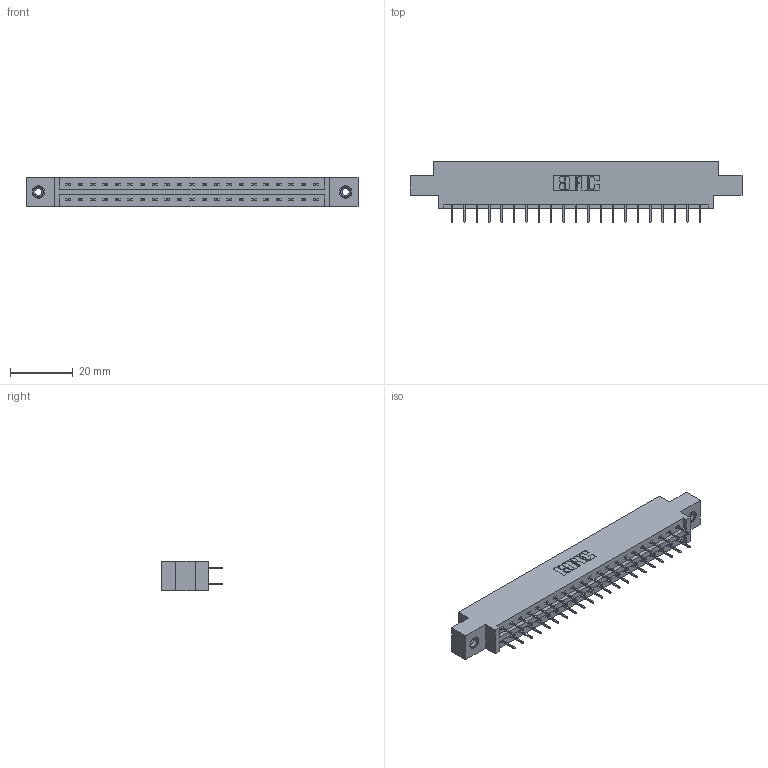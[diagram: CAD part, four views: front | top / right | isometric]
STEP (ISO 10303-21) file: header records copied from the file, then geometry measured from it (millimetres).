
FILE_DESCRIPTION (( 'STEP AP203' ), '1' );
FILE_NAME ('387-042-524-808.STEP', '2018-09-19T22:20:34', ( '' ), ( '' ), 'SwSTEP 2.0', 'SolidWorks 2016', '' );
FILE_SCHEMA (( 'CONFIG_CONTROL_DESIGN' ));
Length unit declared in the file: inch
Products named in the file (4): 387-042-524-808; 337 Part_0.170 Offset - 0.156 Dia-TI; 345-292-001_345-293-124; 345-250-001_345-250-003-102
Assembly tree (45 placements, depth 2):
  387-042-524-808
    337 Part_0.170 Offset - 0.156 Dia-TI
    345-292-001_345-293-124  x42
    345-250-001_345-250-003-102  x2
Bounding box: 106.22 x 19.69 x 9.4 mm (x, y, z)
Volume: 10727.5 mm3; surface area: 11858.4 mm2
Topology: 45 solids, 45 shells, 2614 faces, 7389 edges, 4750 vertices
Faces by surface type: plane 1954, cylinder 644, cone 12, torus 4
Entity records: 20390 total; most frequent: CARTESIAN_POINT 3433, ORIENTED_EDGE 3362, DIRECTION 2991, EDGE_CURVE 1681, LINE 1537, VECTOR 1537, VERTEX_POINT 1112, AXIS2_PLACEMENT_3D 727
